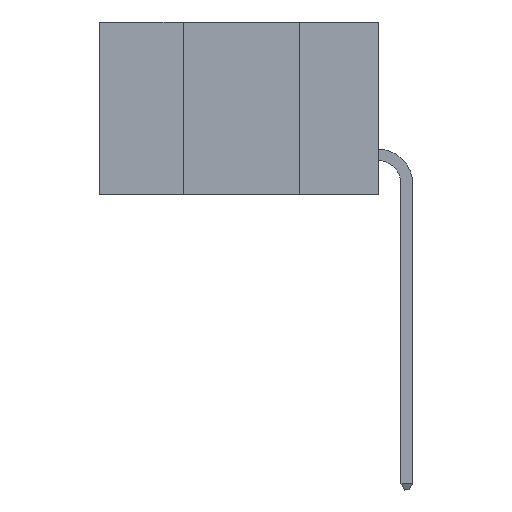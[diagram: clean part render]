
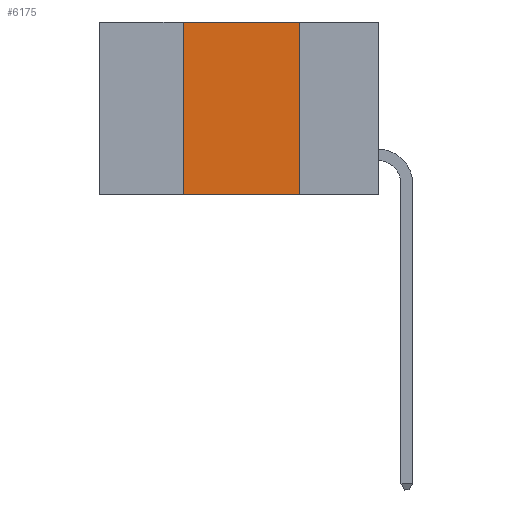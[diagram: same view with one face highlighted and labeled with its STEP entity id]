
A CAD part, left-side view. The second image highlights one B-rep face of the part: STEP entity #6175.
In plain terms, the highlighted planar face has unit normal (-1, 0, 0).
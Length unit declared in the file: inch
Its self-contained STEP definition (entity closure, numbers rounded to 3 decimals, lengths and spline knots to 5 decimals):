
#810 = AXIS2_PLACEMENT_3D ( 'NONE', #21813, #21669, #21667 ) ;
#926 = LINE ( 'NONE', #4056, #5952 ) ;
#1152 = EDGE_CURVE ( 'NONE', #10387, #23391, #926, .T. ) ;
#1898 = VECTOR ( 'NONE', #12820, 39.37008 ) ;
#1907 = CARTESIAN_POINT ( 'NONE',  ( 0., 0.42, -0.37 ) ) ;
#2949 = DIRECTION ( 'NONE',  ( 0., 0., 1. ) ) ;
#3442 = ORIENTED_EDGE ( 'NONE', *, *, #5819, .T. ) ;
#4056 = CARTESIAN_POINT ( 'NONE',  ( 0., 0.42, -0.37 ) ) ;
#5635 = CARTESIAN_POINT ( 'NONE',  ( 0., 0.17, -0.37 ) ) ;
#5819 = EDGE_CURVE ( 'NONE', #10387, #7086, #7509, .T. ) ;
#5952 = VECTOR ( 'NONE', #2949, 39.37008 ) ;
#6175 = ADVANCED_FACE ( 'NONE', ( #23366 ), #21710, .F. ) ;
#6726 = VECTOR ( 'NONE', #11491, 39.37008 ) ;
#7086 = VERTEX_POINT ( 'NONE', #5635 ) ;
#7509 = LINE ( 'NONE', #13178, #1898 ) ;
#10387 = VERTEX_POINT ( 'NONE', #1907 ) ;
#11491 = DIRECTION ( 'NONE',  ( 0., 0., -1. ) ) ;
#11820 = VECTOR ( 'NONE', #15873, 39.37008 ) ;
#12370 = LINE ( 'NONE', #14057, #11820 ) ;
#12820 = DIRECTION ( 'NONE',  ( 0., -1., 0. ) ) ;
#13178 = CARTESIAN_POINT ( 'NONE',  ( 0., 0.6, -0.37 ) ) ;
#13847 = VERTEX_POINT ( 'NONE', #16570 ) ;
#14057 = CARTESIAN_POINT ( 'NONE',  ( 0., 0.6, 0. ) ) ;
#14776 = EDGE_LOOP ( 'NONE', ( #15802, #16353, #17465, #3442 ) ) ;
#15802 = ORIENTED_EDGE ( 'NONE', *, *, #16444, .F. ) ;
#15873 = DIRECTION ( 'NONE',  ( 0., -1., 0. ) ) ;
#16353 = ORIENTED_EDGE ( 'NONE', *, *, #18833, .F. ) ;
#16444 = EDGE_CURVE ( 'NONE', #13847, #7086, #18366, .T. ) ;
#16570 = CARTESIAN_POINT ( 'NONE',  ( 0., 0.17, 0. ) ) ;
#17465 = ORIENTED_EDGE ( 'NONE', *, *, #1152, .F. ) ;
#18366 = LINE ( 'NONE', #22051, #6726 ) ;
#18833 = EDGE_CURVE ( 'NONE', #23391, #13847, #12370, .T. ) ;
#21667 = DIRECTION ( 'NONE',  ( 0., 0., -1. ) ) ;
#21669 = DIRECTION ( 'NONE',  ( 1., 0., 0. ) ) ;
#21710 = PLANE ( 'NONE',  #810 ) ;
#21813 = CARTESIAN_POINT ( 'NONE',  ( 0., 0.6, 0. ) ) ;
#22051 = CARTESIAN_POINT ( 'NONE',  ( 0., 0.17, -0.37 ) ) ;
#23229 = CARTESIAN_POINT ( 'NONE',  ( 0., 0.42, 0. ) ) ;
#23366 = FACE_OUTER_BOUND ( 'NONE', #14776, .T. ) ;
#23391 = VERTEX_POINT ( 'NONE', #23229 ) ;
